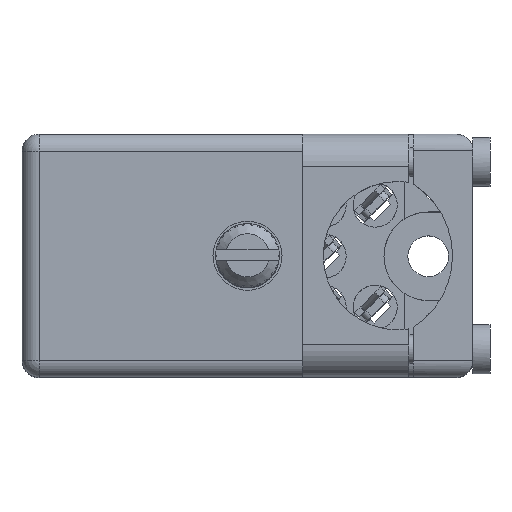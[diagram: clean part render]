
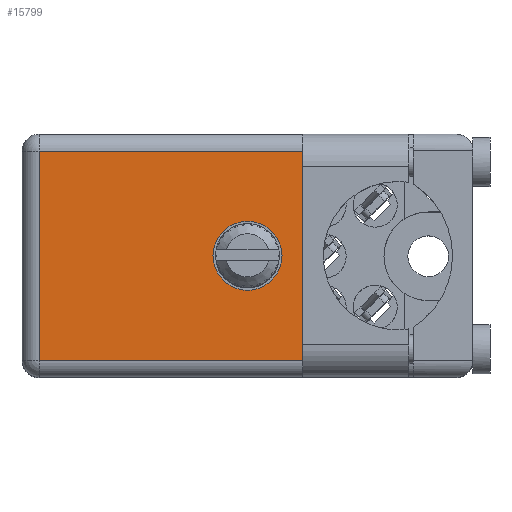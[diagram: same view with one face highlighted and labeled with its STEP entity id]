
A CAD part, top view. The second image highlights one B-rep face of the part: STEP entity #15799.
In plain terms, the highlighted face is planar.
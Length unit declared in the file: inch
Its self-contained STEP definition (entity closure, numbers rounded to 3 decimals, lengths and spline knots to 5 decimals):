
#3918 = CARTESIAN_POINT ( 'NONE',  ( 0.05, 0.906, -0.715 ) ) ;
#6926 = CIRCLE ( 'NONE', #70012, 0.1015 ) ;
#8741 = VERTEX_POINT ( 'NONE', #70552 ) ;
#11641 = AXIS2_PLACEMENT_3D ( 'NONE', #69778, #29234, #27400 ) ;
#12640 = FACE_OUTER_BOUND ( 'NONE', #92703, .T. ) ;
#15799 = ADVANCED_FACE ( 'NONE', ( #12640, #184719 ), #170621, .T. ) ;
#17127 = CARTESIAN_POINT ( 'NONE',  ( 1.15, 0.906, -0.05 ) ) ;
#17509 = VECTOR ( 'NONE', #102850, 39.37008 ) ;
#22271 = ORIENTED_EDGE ( 'NONE', *, *, #112142, .T. ) ;
#22410 = EDGE_CURVE ( 'NONE', #56001, #81847, #6926, .T. ) ;
#24420 = LINE ( 'NONE', #110985, #93359 ) ;
#24458 = DIRECTION ( 'NONE',  ( 0., 1., 0. ) ) ;
#25384 = CARTESIAN_POINT ( 'NONE',  ( 0.6625, 0.906, -0.3575 ) ) ;
#26134 = LINE ( 'NONE', #167301, #179428 ) ;
#27400 = DIRECTION ( 'NONE',  ( 0., 0., 1. ) ) ;
#28254 = DIRECTION ( 'NONE',  ( -1., 0., 0. ) ) ;
#29234 = DIRECTION ( 'NONE',  ( 0., 1., 0. ) ) ;
#36009 = EDGE_CURVE ( 'NONE', #42444, #174923, #67115, .T. ) ;
#38438 = VECTOR ( 'NONE', #45323, 39.37008 ) ;
#39265 = VECTOR ( 'NONE', #28254, 39.37008 ) ;
#39905 = EDGE_CURVE ( 'NONE', #95161, #42444, #171287, .T. ) ;
#41737 = CARTESIAN_POINT ( 'NONE',  ( 0., 0.906, -0.715 ) ) ;
#42444 = VERTEX_POINT ( 'NONE', #150305 ) ;
#42931 = EDGE_CURVE ( 'NONE', #174974, #168013, #24420, .T. ) ;
#45323 = DIRECTION ( 'NONE',  ( 0., 0., 1. ) ) ;
#45484 = LINE ( 'NONE', #126645, #17509 ) ;
#45522 = EDGE_LOOP ( 'NONE', ( #144385, #124193 ) ) ;
#49835 = ORIENTED_EDGE ( 'NONE', *, *, #97094, .T. ) ;
#51628 = DIRECTION ( 'NONE',  ( 1., 0., 0. ) ) ;
#52276 = EDGE_CURVE ( 'NONE', #75494, #8741, #82926, .T. ) ;
#55698 = ORIENTED_EDGE ( 'NONE', *, *, #88766, .F. ) ;
#56001 = VERTEX_POINT ( 'NONE', #152635 ) ;
#63618 = AXIS2_PLACEMENT_3D ( 'NONE', #41737, #99121, #85054 ) ;
#64727 = EDGE_CURVE ( 'NONE', #95161, #168013, #84082, .T. ) ;
#67115 = LINE ( 'NONE', #125344, #156245 ) ;
#68096 = DIRECTION ( 'NONE',  ( 0., 0., 1. ) ) ;
#69778 = CARTESIAN_POINT ( 'NONE',  ( 0.6625, 0.906, -0.3575 ) ) ;
#70012 = AXIS2_PLACEMENT_3D ( 'NONE', #25384, #24458, #137413 ) ;
#70552 = CARTESIAN_POINT ( 'NONE',  ( 0.05, 0.906, -0.665 ) ) ;
#73204 = ORIENTED_EDGE ( 'NONE', *, *, #39905, .T. ) ;
#75494 = VERTEX_POINT ( 'NONE', #133954 ) ;
#81847 = VERTEX_POINT ( 'NONE', #111189 ) ;
#81873 = DIRECTION ( 'NONE',  ( 1., 0., 0. ) ) ;
#82926 = LINE ( 'NONE', #153491, #106325 ) ;
#84082 = LINE ( 'NONE', #154654, #99541 ) ;
#85054 = DIRECTION ( 'NONE',  ( 0., 0., 1. ) ) ;
#88766 = EDGE_CURVE ( 'NONE', #75494, #94142, #45484, .T. ) ;
#91006 = CARTESIAN_POINT ( 'NONE',  ( 1.15, 0.906, -0.6025 ) ) ;
#92703 = EDGE_LOOP ( 'NONE', ( #49835, #167121, #162758, #73204, #179387, #22271, #55698, #148770 ) ) ;
#93359 = VECTOR ( 'NONE', #81873, 39.37008 ) ;
#94142 = VERTEX_POINT ( 'NONE', #91006 ) ;
#95161 = VERTEX_POINT ( 'NONE', #177013 ) ;
#97094 = EDGE_CURVE ( 'NONE', #8741, #174974, #116764, .T. ) ;
#99121 = DIRECTION ( 'NONE',  ( 0., 1., 0. ) ) ;
#99541 = VECTOR ( 'NONE', #68096, 39.37008 ) ;
#102850 = DIRECTION ( 'NONE',  ( 0., 0., 1. ) ) ;
#104795 = CIRCLE ( 'NONE', #11641, 0.1015 ) ;
#106325 = VECTOR ( 'NONE', #184468, 39.37008 ) ;
#110985 = CARTESIAN_POINT ( 'NONE',  ( 1.15, 0.906, -0.05 ) ) ;
#111189 = CARTESIAN_POINT ( 'NONE',  ( 0.6625, 0.906, -0.459 ) ) ;
#112142 = EDGE_CURVE ( 'NONE', #174923, #94142, #26134, .T. ) ;
#116764 = LINE ( 'NONE', #3918, #38438 ) ;
#124193 = ORIENTED_EDGE ( 'NONE', *, *, #131390, .F. ) ;
#124434 = DIRECTION ( 'NONE',  ( 0., 0., -1. ) ) ;
#125344 = CARTESIAN_POINT ( 'NONE',  ( 0.865, 0.906, -0.1125 ) ) ;
#126645 = CARTESIAN_POINT ( 'NONE',  ( 1.15, 0.906, -0.715 ) ) ;
#127982 = CARTESIAN_POINT ( 'NONE',  ( 0.865, 0.906, -0.1125 ) ) ;
#131390 = EDGE_CURVE ( 'NONE', #81847, #56001, #104795, .T. ) ;
#133954 = CARTESIAN_POINT ( 'NONE',  ( 1.15, 0.906, -0.665 ) ) ;
#137413 = DIRECTION ( 'NONE',  ( 0., 0., 1. ) ) ;
#144385 = ORIENTED_EDGE ( 'NONE', *, *, #22410, .F. ) ;
#145956 = CARTESIAN_POINT ( 'NONE',  ( 0.865, 0.906, -0.6025 ) ) ;
#148770 = ORIENTED_EDGE ( 'NONE', *, *, #52276, .T. ) ;
#150305 = CARTESIAN_POINT ( 'NONE',  ( 0.865, 0.906, -0.1125 ) ) ;
#152635 = CARTESIAN_POINT ( 'NONE',  ( 0.6625, 0.906, -0.256 ) ) ;
#153491 = CARTESIAN_POINT ( 'NONE',  ( 0., 0.906, -0.665 ) ) ;
#154654 = CARTESIAN_POINT ( 'NONE',  ( 1.15, 0.906, -0.715 ) ) ;
#156245 = VECTOR ( 'NONE', #124434, 39.37008 ) ;
#162758 = ORIENTED_EDGE ( 'NONE', *, *, #64727, .F. ) ;
#167121 = ORIENTED_EDGE ( 'NONE', *, *, #42931, .T. ) ;
#167301 = CARTESIAN_POINT ( 'NONE',  ( 0.865, 0.906, -0.6025 ) ) ;
#168013 = VERTEX_POINT ( 'NONE', #17127 ) ;
#170621 = PLANE ( 'NONE',  #63618 ) ;
#171287 = LINE ( 'NONE', #127982, #39265 ) ;
#174923 = VERTEX_POINT ( 'NONE', #145956 ) ;
#174974 = VERTEX_POINT ( 'NONE', #180628 ) ;
#177013 = CARTESIAN_POINT ( 'NONE',  ( 1.15, 0.906, -0.1125 ) ) ;
#179387 = ORIENTED_EDGE ( 'NONE', *, *, #36009, .T. ) ;
#179428 = VECTOR ( 'NONE', #51628, 39.37008 ) ;
#180628 = CARTESIAN_POINT ( 'NONE',  ( 0.05, 0.906, -0.05 ) ) ;
#184468 = DIRECTION ( 'NONE',  ( -1., 0., 0. ) ) ;
#184719 = FACE_BOUND ( 'NONE', #45522, .T. ) ;
